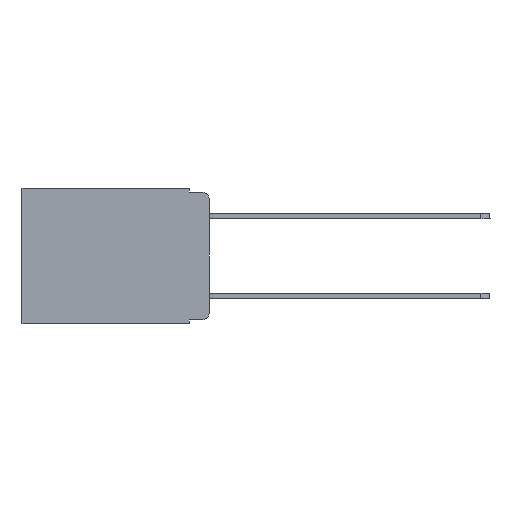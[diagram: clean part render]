
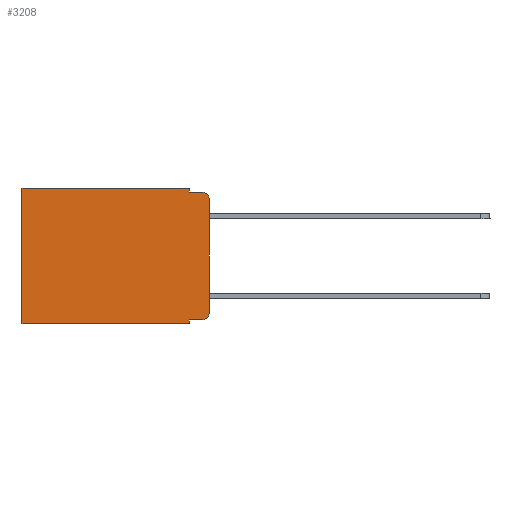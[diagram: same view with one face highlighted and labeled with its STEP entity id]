
A CAD part, left-side view. The second image highlights one B-rep face of the part: STEP entity #3208.
In plain terms, the highlighted planar face has unit normal (-1, 0, 0).
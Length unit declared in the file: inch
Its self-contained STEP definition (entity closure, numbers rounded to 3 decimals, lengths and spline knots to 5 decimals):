
#240 = VECTOR ( 'NONE', #9418, 39.37008 ) ;
#399 = DIRECTION ( 'NONE',  ( -1., 0., 0. ) ) ;
#493 = ORIENTED_EDGE ( 'NONE', *, *, #16184, .T. ) ;
#740 = VERTEX_POINT ( 'NONE', #5203 ) ;
#792 = ORIENTED_EDGE ( 'NONE', *, *, #6587, .T. ) ;
#927 = AXIS2_PLACEMENT_3D ( 'NONE', #17506, #5921, #10237 ) ;
#971 = DIRECTION ( 'NONE',  ( 0., 0., -1. ) ) ;
#1042 = EDGE_CURVE ( 'NONE', #17653, #740, #8727, .T. ) ;
#1052 = CARTESIAN_POINT ( 'NONE',  ( 0.298, 0.02, -0.333 ) ) ;
#1404 = DIRECTION ( 'NONE',  ( 0., 0., -1. ) ) ;
#1579 = CARTESIAN_POINT ( 'NONE',  ( 0.298, 0.02, -0.313 ) ) ;
#1932 = VECTOR ( 'NONE', #11960, 39.37008 ) ;
#2126 = ORIENTED_EDGE ( 'NONE', *, *, #6636, .F. ) ;
#2192 = VERTEX_POINT ( 'NONE', #1052 ) ;
#2388 = CIRCLE ( 'NONE', #17502, 0.02 ) ;
#2427 = ORIENTED_EDGE ( 'NONE', *, *, #18170, .T. ) ;
#2546 = CIRCLE ( 'NONE', #7487, 0.02 ) ;
#2637 = CARTESIAN_POINT ( 'NONE',  ( 0.298, 0.02, -0.01 ) ) ;
#2822 = ORIENTED_EDGE ( 'NONE', *, *, #7348, .F. ) ;
#2913 = DIRECTION ( 'NONE',  ( 0., 0., -1. ) ) ;
#3208 = ADVANCED_FACE ( 'NONE', ( #13322 ), #4461, .F. ) ;
#3309 = VECTOR ( 'NONE', #6310, 39.37008 ) ;
#3320 = VECTOR ( 'NONE', #4720, 39.37008 ) ;
#3402 = CARTESIAN_POINT ( 'NONE',  ( 0.298, 0., 0. ) ) ;
#3795 = CARTESIAN_POINT ( 'NONE',  ( 0.298, 0., 0. ) ) ;
#4461 = PLANE ( 'NONE',  #927 ) ;
#4720 = DIRECTION ( 'NONE',  ( 0., 0., -1. ) ) ;
#4827 = EDGE_CURVE ( 'NONE', #11396, #10952, #15784, .T. ) ;
#5203 = CARTESIAN_POINT ( 'NONE',  ( 0.298, 0.473, -0.343 ) ) ;
#5363 = VECTOR ( 'NONE', #7008, 39.37008 ) ;
#5921 = DIRECTION ( 'NONE',  ( 1., 0., 0. ) ) ;
#6030 = VERTEX_POINT ( 'NONE', #17663 ) ;
#6310 = DIRECTION ( 'NONE',  ( 0., 0., -1. ) ) ;
#6587 = EDGE_CURVE ( 'NONE', #8618, #740, #13228, .T. ) ;
#6636 = EDGE_CURVE ( 'NONE', #10857, #6030, #14583, .T. ) ;
#7008 = DIRECTION ( 'NONE',  ( 0., -1., 0. ) ) ;
#7117 = ORIENTED_EDGE ( 'NONE', *, *, #1042, .F. ) ;
#7280 = EDGE_CURVE ( 'NONE', #10857, #10952, #2388, .T. ) ;
#7348 = EDGE_CURVE ( 'NONE', #10706, #11396, #15681, .T. ) ;
#7487 = AXIS2_PLACEMENT_3D ( 'NONE', #1579, #399, #14613 ) ;
#8618 = VERTEX_POINT ( 'NONE', #13823 ) ;
#8727 = LINE ( 'NONE', #16275, #1932 ) ;
#9418 = DIRECTION ( 'NONE',  ( 0., -1., 0. ) ) ;
#9427 = LINE ( 'NONE', #11906, #3320 ) ;
#9597 = CARTESIAN_POINT ( 'NONE',  ( 0.298, 0.051, 0. ) ) ;
#9987 = ORIENTED_EDGE ( 'NONE', *, *, #7280, .T. ) ;
#10237 = DIRECTION ( 'NONE',  ( 0., 0., -1. ) ) ;
#10631 = CARTESIAN_POINT ( 'NONE',  ( 0.298, 0.051, -0.333 ) ) ;
#10706 = VERTEX_POINT ( 'NONE', #11959 ) ;
#10781 = CARTESIAN_POINT ( 'NONE',  ( 0.298, 0.051, -0.01 ) ) ;
#10857 = VERTEX_POINT ( 'NONE', #10935 ) ;
#10935 = CARTESIAN_POINT ( 'NONE',  ( 0.298, 0., -0.03 ) ) ;
#10952 = VERTEX_POINT ( 'NONE', #2637 ) ;
#11396 = VERTEX_POINT ( 'NONE', #10781 ) ;
#11906 = CARTESIAN_POINT ( 'NONE',  ( 0.298, 0.051, 0. ) ) ;
#11959 = CARTESIAN_POINT ( 'NONE',  ( 0.298, 0.051, 0. ) ) ;
#11960 = DIRECTION ( 'NONE',  ( 0., 1., 0. ) ) ;
#12058 = ORIENTED_EDGE ( 'NONE', *, *, #4827, .F. ) ;
#12091 = VECTOR ( 'NONE', #13761, 39.37008 ) ;
#12329 = VECTOR ( 'NONE', #2913, 39.37008 ) ;
#12639 = ORIENTED_EDGE ( 'NONE', *, *, #16828, .F. ) ;
#12963 = VECTOR ( 'NONE', #971, 39.37008 ) ;
#13001 = LINE ( 'NONE', #3795, #12091 ) ;
#13228 = LINE ( 'NONE', #16222, #12329 ) ;
#13257 = LINE ( 'NONE', #16427, #240 ) ;
#13263 = DIRECTION ( 'NONE',  ( -1., 0., 0. ) ) ;
#13322 = FACE_OUTER_BOUND ( 'NONE', #17987, .T. ) ;
#13439 = CARTESIAN_POINT ( 'NONE',  ( 0.298, 0.02, -0.03 ) ) ;
#13761 = DIRECTION ( 'NONE',  ( 0., 1., 0. ) ) ;
#13823 = CARTESIAN_POINT ( 'NONE',  ( 0.298, 0.473, 0. ) ) ;
#14362 = EDGE_CURVE ( 'NONE', #2192, #6030, #2546, .T. ) ;
#14583 = LINE ( 'NONE', #3402, #3309 ) ;
#14613 = DIRECTION ( 'NONE',  ( 0., 0., -1. ) ) ;
#15414 = CARTESIAN_POINT ( 'NONE',  ( 0.298, 0.051, -0.343 ) ) ;
#15681 = LINE ( 'NONE', #9597, #12963 ) ;
#15784 = LINE ( 'NONE', #18352, #5363 ) ;
#15837 = VERTEX_POINT ( 'NONE', #10631 ) ;
#15875 = ORIENTED_EDGE ( 'NONE', *, *, #14362, .T. ) ;
#16184 = EDGE_CURVE ( 'NONE', #15837, #2192, #13257, .T. ) ;
#16222 = CARTESIAN_POINT ( 'NONE',  ( 0.298, 0.473, 0. ) ) ;
#16275 = CARTESIAN_POINT ( 'NONE',  ( 0.298, 0., -0.343 ) ) ;
#16427 = CARTESIAN_POINT ( 'NONE',  ( 0.298, 0.051, -0.333 ) ) ;
#16828 = EDGE_CURVE ( 'NONE', #15837, #17653, #9427, .T. ) ;
#17502 = AXIS2_PLACEMENT_3D ( 'NONE', #13439, #13263, #1404 ) ;
#17506 = CARTESIAN_POINT ( 'NONE',  ( 0.298, 0., 0. ) ) ;
#17653 = VERTEX_POINT ( 'NONE', #15414 ) ;
#17663 = CARTESIAN_POINT ( 'NONE',  ( 0.298, 0., -0.313 ) ) ;
#17987 = EDGE_LOOP ( 'NONE', ( #2126, #9987, #12058, #2822, #2427, #792, #7117, #12639, #493, #15875 ) ) ;
#18170 = EDGE_CURVE ( 'NONE', #10706, #8618, #13001, .T. ) ;
#18352 = CARTESIAN_POINT ( 'NONE',  ( 0.298, 0.051, -0.01 ) ) ;
